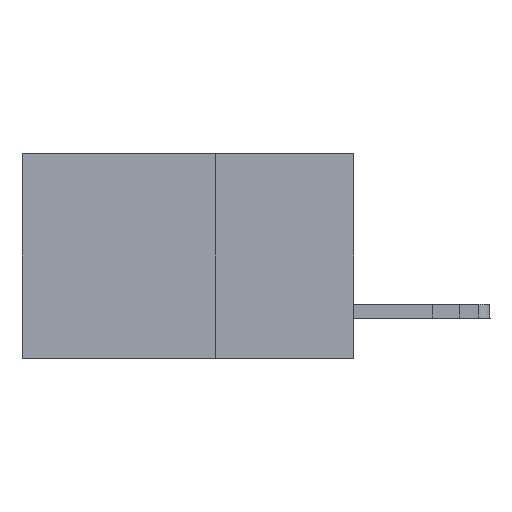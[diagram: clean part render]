
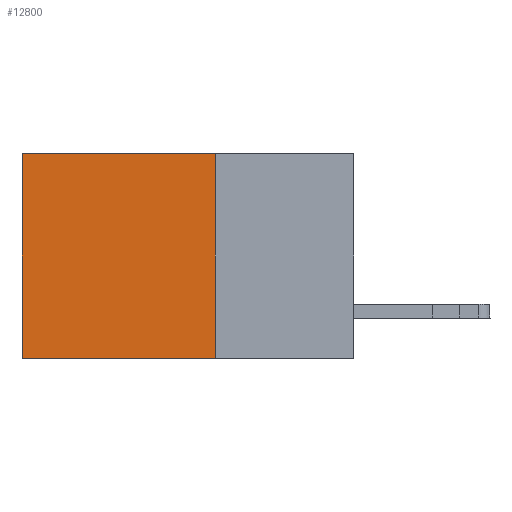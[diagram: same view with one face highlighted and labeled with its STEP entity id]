
A CAD part, left-side view. The second image highlights one B-rep face of the part: STEP entity #12800.
In plain terms, the highlighted planar face has unit normal (-1, 0, 0).
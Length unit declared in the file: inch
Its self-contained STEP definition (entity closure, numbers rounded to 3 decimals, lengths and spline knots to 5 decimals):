
#480 = LINE ( 'NONE', #9714, #16372 ) ;
#1300 = VERTEX_POINT ( 'NONE', #2634 ) ;
#1890 = VERTEX_POINT ( 'NONE', #17205 ) ;
#2233 = PLANE ( 'NONE',  #7257 ) ;
#2634 = CARTESIAN_POINT ( 'NONE',  ( 0.2875, 0.25, 0. ) ) ;
#3651 = EDGE_CURVE ( 'NONE', #1890, #18571, #21400, .T. ) ;
#4114 = EDGE_LOOP ( 'NONE', ( #10836, #23252, #26427, #14176 ) ) ;
#4996 = LINE ( 'NONE', #19523, #20917 ) ;
#6473 = DIRECTION ( 'NONE',  ( 0., 0., -1. ) ) ;
#7257 = AXIS2_PLACEMENT_3D ( 'NONE', #16691, #18824, #6473 ) ;
#7422 = EDGE_CURVE ( 'NONE', #1300, #19094, #21029, .T. ) ;
#8569 = CARTESIAN_POINT ( 'NONE',  ( 0.2875, 0.6, -0.37 ) ) ;
#9714 = CARTESIAN_POINT ( 'NONE',  ( 0.2875, 0.25, 0. ) ) ;
#10025 = FACE_OUTER_BOUND ( 'NONE', #4114, .T. ) ;
#10506 = VECTOR ( 'NONE', #24941, 39.37008 ) ;
#10836 = ORIENTED_EDGE ( 'NONE', *, *, #25802, .T. ) ;
#12294 = CARTESIAN_POINT ( 'NONE',  ( 0.2875, 0.25, 0. ) ) ;
#12800 = ADVANCED_FACE ( 'NONE', ( #10025 ), #2233, .F. ) ;
#14176 = ORIENTED_EDGE ( 'NONE', *, *, #7422, .T. ) ;
#14382 = CARTESIAN_POINT ( 'NONE',  ( 0.2875, 0.25, -0.37 ) ) ;
#15030 = VECTOR ( 'NONE', #16492, 39.37008 ) ;
#16372 = VECTOR ( 'NONE', #24386, 39.37008 ) ;
#16492 = DIRECTION ( 'NONE',  ( 0., 1., 0. ) ) ;
#16691 = CARTESIAN_POINT ( 'NONE',  ( 0.2875, 0.25, 0. ) ) ;
#17205 = CARTESIAN_POINT ( 'NONE',  ( 0.2875, 0.25, -0.37 ) ) ;
#18571 = VERTEX_POINT ( 'NONE', #8569 ) ;
#18824 = DIRECTION ( 'NONE',  ( 1., 0., 0. ) ) ;
#19094 = VERTEX_POINT ( 'NONE', #21868 ) ;
#19523 = CARTESIAN_POINT ( 'NONE',  ( 0.2875, 0.6, 0. ) ) ;
#20917 = VECTOR ( 'NONE', #23808, 39.37008 ) ;
#21029 = LINE ( 'NONE', #12294, #10506 ) ;
#21400 = LINE ( 'NONE', #14382, #15030 ) ;
#21868 = CARTESIAN_POINT ( 'NONE',  ( 0.2875, 0.6, 0. ) ) ;
#22958 = EDGE_CURVE ( 'NONE', #1300, #1890, #480, .T. ) ;
#23252 = ORIENTED_EDGE ( 'NONE', *, *, #3651, .F. ) ;
#23808 = DIRECTION ( 'NONE',  ( 0., 0., -1. ) ) ;
#24386 = DIRECTION ( 'NONE',  ( 0., 0., -1. ) ) ;
#24941 = DIRECTION ( 'NONE',  ( 0., 1., 0. ) ) ;
#25802 = EDGE_CURVE ( 'NONE', #19094, #18571, #4996, .T. ) ;
#26427 = ORIENTED_EDGE ( 'NONE', *, *, #22958, .F. ) ;
